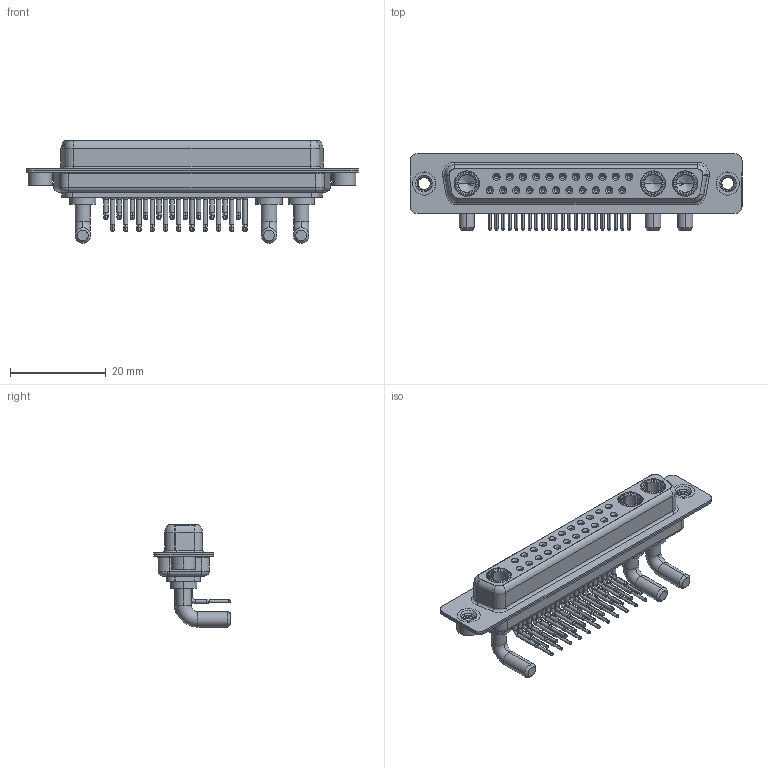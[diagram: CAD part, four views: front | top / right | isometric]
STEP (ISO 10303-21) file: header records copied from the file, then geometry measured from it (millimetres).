
FILE_DESCRIPTION (( 'STEP AP203' ), '1' );
FILE_NAME ('630-25W3240-3TA.STEP', '2022-06-07T03:00:47', ( '' ), ( '' ), 'SwSTEP 2.0', 'SolidWorks 2020', '' );
FILE_SCHEMA (( 'CONFIG_CONTROL_DESIGN' ));
Length unit declared in the file: millimetre
Products named in the file (8): 630Combo Housing_25W3; 630-25W3240-3TA; 630Combo Contact Row 2; 630Combo Shell Front_37 Contacts; 630Combo Shell Rear_37 Contacts; 630Combo Contact Row 1; 630Combo Threaded Rivet_A; Power Socket_30A RA
Assembly tree (30 placements, depth 2):
  630-25W3240-3TA
    630Combo Housing_25W3
    630Combo Shell Front_37 Contacts
    630Combo Shell Rear_37 Contacts
    630Combo Threaded Rivet_A  x2
    Power Socket_30A RA  x3
    630Combo Contact Row 1  x11
    630Combo Contact Row 2  x11
Bounding box: 69.4 x 16 x 21.4 mm (x, y, z)
Volume: 5753.5 mm3; surface area: 12774 mm2
Topology: 33 solids, 33 shells, 1673 faces, 4259 edges, 2688 vertices
Faces by surface type: cylinder 716, plane 484, cone 301, bspline 97, torus 75
Entity records: 23725 total; most frequent: CARTESIAN_POINT 5477, DIRECTION 3838, ORIENTED_EDGE 3290, EDGE_CURVE 1645, AXIS2_PLACEMENT_3D 1602, VERTEX_POINT 1050, CIRCLE 884, EDGE_LOOP 847
